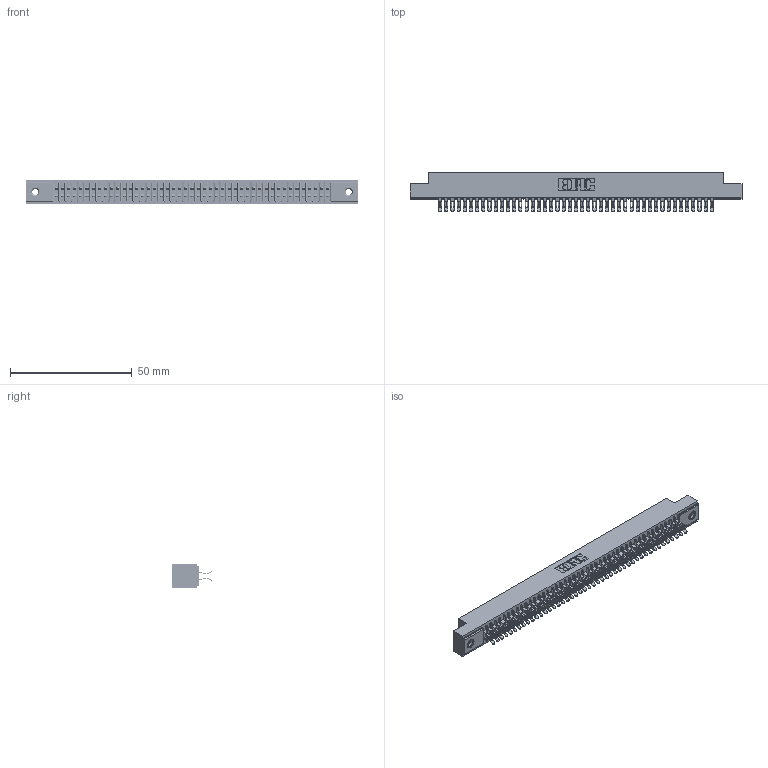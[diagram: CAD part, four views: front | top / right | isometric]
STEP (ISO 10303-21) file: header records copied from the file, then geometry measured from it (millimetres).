
FILE_DESCRIPTION (( 'STEP AP203' ), '1' );
FILE_NAME ('341-090-555-207.STEP', '2018-08-08T00:14:30', ( '' ), ( '' ), 'SwSTEP 2.0', 'SolidWorks 2016', '' );
FILE_SCHEMA (( 'CONFIG_CONTROL_DESIGN' ));
Length unit declared in the file: inch
Products named in the file (4): 345-250-001_345-250-005-103; 341-090-555-207; 341 Part_.156 (3.96) Dia Mounting Holes; 341-292-001_341-292-155
Assembly tree (93 placements, depth 2):
  341-090-555-207
    341 Part_.156 (3.96) Dia Mounting Holes
    341-292-001_341-292-155  x90
    345-250-001_345-250-005-103  x2
Bounding box: 136.53 x 16.31 x 10.16 mm (x, y, z)
Volume: 10185.2 mm3; surface area: 18944.5 mm2
Topology: 93 solids, 93 shells, 7196 faces, 21467 edges, 13970 vertices
Faces by surface type: plane 3880, cylinder 3120, sphere 92, torus 92, cone 12
Entity records: 55715 total; most frequent: CARTESIAN_POINT 9260, ORIENTED_EDGE 9186, DIRECTION 8985, EDGE_CURVE 4593, VECTOR 3695, LINE 3695, VERTEX_POINT 2904, AXIS2_PLACEMENT_3D 2645
